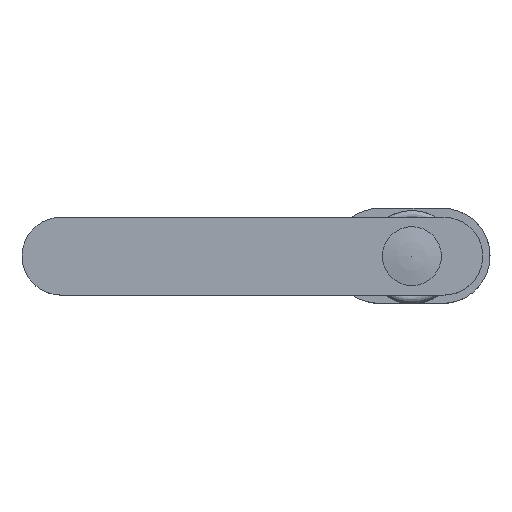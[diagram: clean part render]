
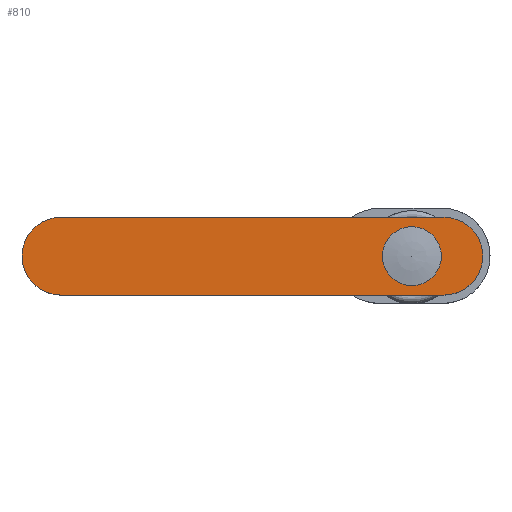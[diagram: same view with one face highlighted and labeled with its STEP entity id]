
A CAD part, top view. The second image highlights one B-rep face of the part: STEP entity #810.
In plain terms, the highlighted planar face has unit normal (0, 0, 1).
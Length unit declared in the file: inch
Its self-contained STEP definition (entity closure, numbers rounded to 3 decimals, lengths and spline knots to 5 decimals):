
#98=FACE_BOUND('',#207,.T.);
#99=FACE_BOUND('',#208,.T.);
#109=CIRCLE('',#869,0.0935);
#111=CIRCLE('',#873,0.12343);
#112=CIRCLE('',#874,0.12343);
#207=EDGE_LOOP('',(#564));
#208=EDGE_LOOP('',(#565,#566,#567,#568));
#273=LINE('',#1223,#315);
#274=LINE('',#1227,#316);
#315=VECTOR('',#989,1.21535);
#316=VECTOR('',#992,1.21535);
#353=VERTEX_POINT('',#1209);
#358=VERTEX_POINT('',#1221);
#359=VERTEX_POINT('',#1222);
#360=VERTEX_POINT('',#1224);
#361=VERTEX_POINT('',#1226);
#437=EDGE_CURVE('',#353,#353,#109,.T.);
#442=EDGE_CURVE('',#358,#359,#273,.T.);
#443=EDGE_CURVE('',#359,#360,#111,.T.);
#444=EDGE_CURVE('',#360,#361,#274,.T.);
#445=EDGE_CURVE('',#361,#358,#112,.T.);
#564=ORIENTED_EDGE('',*,*,#437,.T.);
#565=ORIENTED_EDGE('',*,*,#442,.T.);
#566=ORIENTED_EDGE('',*,*,#443,.T.);
#567=ORIENTED_EDGE('',*,*,#444,.T.);
#568=ORIENTED_EDGE('',*,*,#445,.T.);
#784=PLANE('',#872);
#810=ADVANCED_FACE('',(#98,#99),#784,.T.);
#869=AXIS2_PLACEMENT_3D('',#1210,#978,#979);
#872=AXIS2_PLACEMENT_3D('',#1220,#987,#988);
#873=AXIS2_PLACEMENT_3D('',#1225,#990,#991);
#874=AXIS2_PLACEMENT_3D('',#1228,#993,#994);
#978=DIRECTION('center_axis',(0.,0.,-1.));
#979=DIRECTION('ref_axis',(1.,0.,0.));
#987=DIRECTION('center_axis',(0.,0.,1.));
#988=DIRECTION('ref_axis',(1.,0.,0.));
#989=DIRECTION('',(1.,0.,0.));
#990=DIRECTION('center_axis',(0.,0.,1.));
#991=DIRECTION('ref_axis',(0.,-1.,0.));
#992=DIRECTION('',(-1.,0.,0.));
#993=DIRECTION('center_axis',(0.,0.,1.));
#994=DIRECTION('ref_axis',(0.,1.,0.));
#1209=CARTESIAN_POINT('',(0.4126,0.,0.07874));
#1210=CARTESIAN_POINT('Origin',(0.5061,0.,
0.07874));
#1220=CARTESIAN_POINT('Origin',(0.,0.,0.07874));
#1221=CARTESIAN_POINT('',(-0.60768,-0.12343,0.07874));
#1222=CARTESIAN_POINT('',(0.60768,-0.12343,0.07874));
#1223=CARTESIAN_POINT('',(-0.60768,-0.12343,0.07874));
#1224=CARTESIAN_POINT('',(0.60768,0.12343,0.07874));
#1225=CARTESIAN_POINT('Origin',(0.60768,0.,
0.07874));
#1226=CARTESIAN_POINT('',(-0.60768,0.12343,0.07874));
#1227=CARTESIAN_POINT('',(0.60768,0.12343,0.07874));
#1228=CARTESIAN_POINT('Origin',(-0.60768,0.,
0.07874));
